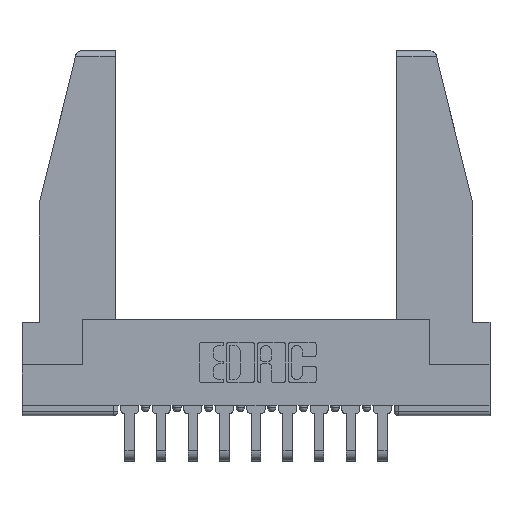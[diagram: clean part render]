
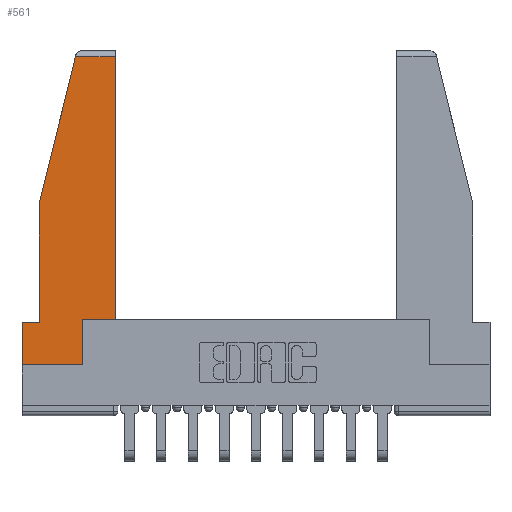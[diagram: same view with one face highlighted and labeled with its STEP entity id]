
A CAD part, top view. The second image highlights one B-rep face of the part: STEP entity #561.
In plain terms, the highlighted planar face has unit normal (0, 0, 1).
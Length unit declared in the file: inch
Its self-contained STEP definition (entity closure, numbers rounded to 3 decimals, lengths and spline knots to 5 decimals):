
#255 = ORIENTED_EDGE ( 'NONE', *, *, #1247, .T. ) ;
#289 = DIRECTION ( 'NONE',  ( 0., -1., 0. ) ) ;
#561 = ADVANCED_FACE ( 'NONE', ( #13163 ), #9416, .T. ) ;
#564 = CARTESIAN_POINT ( 'NONE',  ( 0., 0.21, 0. ) ) ;
#850 = VERTEX_POINT ( 'NONE', #8522 ) ;
#877 = DIRECTION ( 'NONE',  ( 0., -1., 0. ) ) ;
#897 = CARTESIAN_POINT ( 'NONE',  ( 0., 0., 0. ) ) ;
#1247 = EDGE_CURVE ( 'NONE', #10072, #4884, #3474, .T. ) ;
#1870 = VECTOR ( 'NONE', #4655, 39.37008 ) ;
#1886 = LINE ( 'NONE', #6828, #13190 ) ;
#2032 = DIRECTION ( 'NONE',  ( -0.239, -0.971, 0. ) ) ;
#2194 = VECTOR ( 'NONE', #15183, 39.37008 ) ;
#2202 = EDGE_CURVE ( 'NONE', #4884, #13668, #4336, .T. ) ;
#2261 = ORIENTED_EDGE ( 'NONE', *, *, #2202, .T. ) ;
#2369 = VECTOR ( 'NONE', #9304, 39.37008 ) ;
#2398 = DIRECTION ( 'NONE',  ( -1., 0., 0. ) ) ;
#2625 = ORIENTED_EDGE ( 'NONE', *, *, #4493, .T. ) ;
#2652 = AXIS2_PLACEMENT_3D ( 'NONE', #3307, #10714, #5733 ) ;
#3119 = VECTOR ( 'NONE', #2398, 39.37008 ) ;
#3307 = CARTESIAN_POINT ( 'NONE',  ( 0., 0., 0. ) ) ;
#3474 = LINE ( 'NONE', #4666, #5316 ) ;
#3528 = VERTEX_POINT ( 'NONE', #5311 ) ;
#4311 = EDGE_CURVE ( 'NONE', #3528, #5381, #5011, .T. ) ;
#4336 = LINE ( 'NONE', #15795, #1870 ) ;
#4481 = CARTESIAN_POINT ( 'NONE',  ( 0., 0.21, 0. ) ) ;
#4493 = EDGE_CURVE ( 'NONE', #13455, #10072, #14485, .T. ) ;
#4655 = DIRECTION ( 'NONE',  ( 1., 0., 0. ) ) ;
#4666 = CARTESIAN_POINT ( 'NONE',  ( 0.297, 0., 0. ) ) ;
#4675 = VECTOR ( 'NONE', #877, 39.37008 ) ;
#4884 = VERTEX_POINT ( 'NONE', #11388 ) ;
#4984 = LINE ( 'NONE', #13620, #3119 ) ;
#5011 = LINE ( 'NONE', #11447, #8762 ) ;
#5178 = CARTESIAN_POINT ( 'NONE',  ( 0.461, 0.223, 0. ) ) ;
#5282 = ORIENTED_EDGE ( 'NONE', *, *, #7109, .T. ) ;
#5311 = CARTESIAN_POINT ( 'NONE',  ( 0.086, 0.8, 0. ) ) ;
#5316 = VECTOR ( 'NONE', #6951, 39.37008 ) ;
#5381 = VERTEX_POINT ( 'NONE', #10213 ) ;
#5733 = DIRECTION ( 'NONE',  ( 1., 0., 0. ) ) ;
#5780 = DIRECTION ( 'NONE',  ( 1., 0., 0. ) ) ;
#6011 = EDGE_CURVE ( 'NONE', #13668, #15588, #7543, .T. ) ;
#6828 = CARTESIAN_POINT ( 'NONE',  ( 0.271, 1.55, 0. ) ) ;
#6951 = DIRECTION ( 'NONE',  ( 0., 1., 0. ) ) ;
#7109 = EDGE_CURVE ( 'NONE', #850, #3528, #1886, .T. ) ;
#7543 = LINE ( 'NONE', #5178, #2194 ) ;
#7767 = CARTESIAN_POINT ( 'NONE',  ( 0.297, 0., 0. ) ) ;
#8412 = VERTEX_POINT ( 'NONE', #4481 ) ;
#8522 = CARTESIAN_POINT ( 'NONE',  ( 0.2636, 1.52, 0. ) ) ;
#8762 = VECTOR ( 'NONE', #289, 39.37008 ) ;
#9304 = DIRECTION ( 'NONE',  ( -1., 0., 0. ) ) ;
#9416 = PLANE ( 'NONE',  #2652 ) ;
#9906 = EDGE_CURVE ( 'NONE', #15588, #850, #4984, .T. ) ;
#10072 = VERTEX_POINT ( 'NONE', #7767 ) ;
#10213 = CARTESIAN_POINT ( 'NONE',  ( 0.086, 0.21, 0. ) ) ;
#10541 = CARTESIAN_POINT ( 'NONE',  ( 0., 0.21, 0. ) ) ;
#10590 = ORIENTED_EDGE ( 'NONE', *, *, #6011, .T. ) ;
#10685 = EDGE_CURVE ( 'NONE', #8412, #13455, #14164, .T. ) ;
#10714 = DIRECTION ( 'NONE',  ( 0., 0., 1. ) ) ;
#11388 = CARTESIAN_POINT ( 'NONE',  ( 0.297, 0.223, 0. ) ) ;
#11447 = CARTESIAN_POINT ( 'NONE',  ( 0.086, 0.8, 0. ) ) ;
#11634 = CARTESIAN_POINT ( 'NONE',  ( 0., 0., 0. ) ) ;
#12297 = EDGE_LOOP ( 'NONE', ( #10590, #14488, #5282, #14967, #15747, #14621, #2625, #255, #2261 ) ) ;
#12813 = CARTESIAN_POINT ( 'NONE',  ( 0.461, 1.52, 0. ) ) ;
#13163 = FACE_OUTER_BOUND ( 'NONE', #12297, .T. ) ;
#13190 = VECTOR ( 'NONE', #2032, 39.37008 ) ;
#13455 = VERTEX_POINT ( 'NONE', #11634 ) ;
#13620 = CARTESIAN_POINT ( 'NONE',  ( 0., 1.52, 0. ) ) ;
#13668 = VERTEX_POINT ( 'NONE', #15441 ) ;
#13899 = EDGE_CURVE ( 'NONE', #5381, #8412, #14030, .T. ) ;
#14030 = LINE ( 'NONE', #10541, #2369 ) ;
#14163 = VECTOR ( 'NONE', #5780, 39.37008 ) ;
#14164 = LINE ( 'NONE', #564, #4675 ) ;
#14485 = LINE ( 'NONE', #897, #14163 ) ;
#14488 = ORIENTED_EDGE ( 'NONE', *, *, #9906, .T. ) ;
#14621 = ORIENTED_EDGE ( 'NONE', *, *, #10685, .T. ) ;
#14967 = ORIENTED_EDGE ( 'NONE', *, *, #4311, .T. ) ;
#15183 = DIRECTION ( 'NONE',  ( 0., 1., 0. ) ) ;
#15441 = CARTESIAN_POINT ( 'NONE',  ( 0.461, 0.223, 0. ) ) ;
#15588 = VERTEX_POINT ( 'NONE', #12813 ) ;
#15747 = ORIENTED_EDGE ( 'NONE', *, *, #13899, .T. ) ;
#15795 = CARTESIAN_POINT ( 'NONE',  ( 0.297, 0.223, 0. ) ) ;
